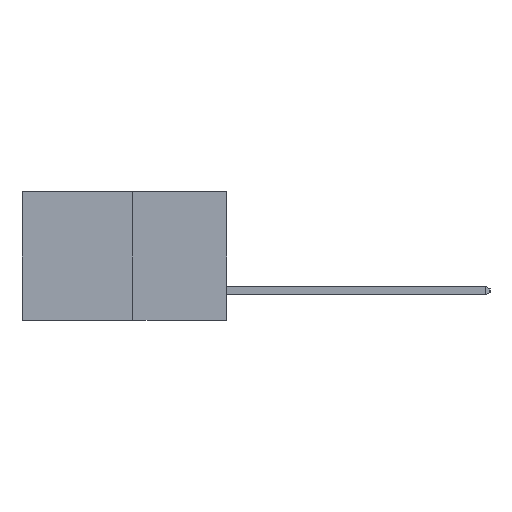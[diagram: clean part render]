
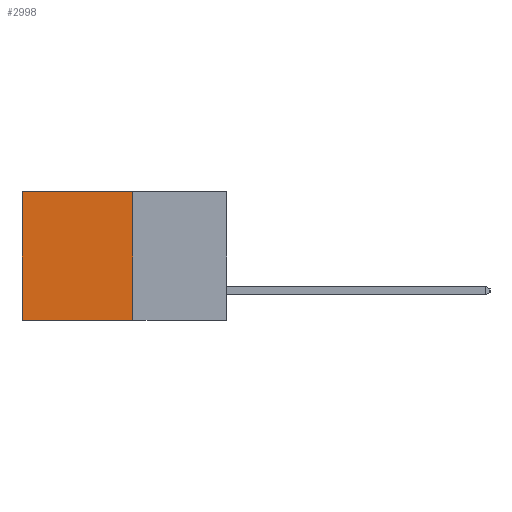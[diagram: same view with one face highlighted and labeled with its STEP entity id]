
A CAD part, left-side view. The second image highlights one B-rep face of the part: STEP entity #2998.
In plain terms, the highlighted planar face has unit normal (-1, 0, 0).
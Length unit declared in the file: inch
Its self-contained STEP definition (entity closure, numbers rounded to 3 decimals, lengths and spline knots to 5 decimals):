
#231 = CARTESIAN_POINT ( 'NONE',  ( 0.277, 0.27, 0. ) ) ;
#732 = ORIENTED_EDGE ( 'NONE', *, *, #22533, .F. ) ;
#1588 = CARTESIAN_POINT ( 'NONE',  ( 0.277, 0.27, -0.37 ) ) ;
#2998 = ADVANCED_FACE ( 'NONE', ( #7797 ), #10292, .F. ) ;
#3006 = AXIS2_PLACEMENT_3D ( 'NONE', #10523, #10254, #10234 ) ;
#3180 = VECTOR ( 'NONE', #19381, 39.37008 ) ;
#3549 = VERTEX_POINT ( 'NONE', #3585 ) ;
#3585 = CARTESIAN_POINT ( 'NONE',  ( 0.277, 0.59, 0. ) ) ;
#5414 = CARTESIAN_POINT ( 'NONE',  ( 0.277, 0.27, -0.37 ) ) ;
#6437 = LINE ( 'NONE', #14544, #15735 ) ;
#6681 = DIRECTION ( 'NONE',  ( 0., 0., -1. ) ) ;
#7194 = ORIENTED_EDGE ( 'NONE', *, *, #7516, .T. ) ;
#7516 = EDGE_CURVE ( 'NONE', #9848, #3549, #8600, .T. ) ;
#7797 = FACE_OUTER_BOUND ( 'NONE', #12660, .T. ) ;
#7985 = LINE ( 'NONE', #5414, #3180 ) ;
#8600 = LINE ( 'NONE', #231, #24939 ) ;
#9848 = VERTEX_POINT ( 'NONE', #9856 ) ;
#9856 = CARTESIAN_POINT ( 'NONE',  ( 0.277, 0.27, 0. ) ) ;
#10234 = DIRECTION ( 'NONE',  ( 0., 0., -1. ) ) ;
#10254 = DIRECTION ( 'NONE',  ( 1., 0., 0. ) ) ;
#10292 = PLANE ( 'NONE',  #3006 ) ;
#10476 = ORIENTED_EDGE ( 'NONE', *, *, #11462, .F. ) ;
#10523 = CARTESIAN_POINT ( 'NONE',  ( 0.277, 0.27, -0.37 ) ) ;
#11462 = EDGE_CURVE ( 'NONE', #15281, #13628, #7985, .T. ) ;
#12660 = EDGE_LOOP ( 'NONE', ( #22230, #10476, #732, #7194 ) ) ;
#13037 = CARTESIAN_POINT ( 'NONE',  ( 0.277, 0.27, -0.37 ) ) ;
#13628 = VERTEX_POINT ( 'NONE', #22788 ) ;
#14544 = CARTESIAN_POINT ( 'NONE',  ( 0.277, 0.59, -0.37 ) ) ;
#15281 = VERTEX_POINT ( 'NONE', #1588 ) ;
#15735 = VECTOR ( 'NONE', #6681, 39.37008 ) ;
#16547 = VECTOR ( 'NONE', #22899, 39.37008 ) ;
#18340 = DIRECTION ( 'NONE',  ( 0., 1., 0. ) ) ;
#19381 = DIRECTION ( 'NONE',  ( 0., 1., 0. ) ) ;
#21788 = LINE ( 'NONE', #13037, #16547 ) ;
#22230 = ORIENTED_EDGE ( 'NONE', *, *, #25023, .T. ) ;
#22533 = EDGE_CURVE ( 'NONE', #9848, #15281, #21788, .T. ) ;
#22788 = CARTESIAN_POINT ( 'NONE',  ( 0.277, 0.59, -0.37 ) ) ;
#22899 = DIRECTION ( 'NONE',  ( 0., 0., -1. ) ) ;
#24939 = VECTOR ( 'NONE', #18340, 39.37008 ) ;
#25023 = EDGE_CURVE ( 'NONE', #3549, #13628, #6437, .T. ) ;
